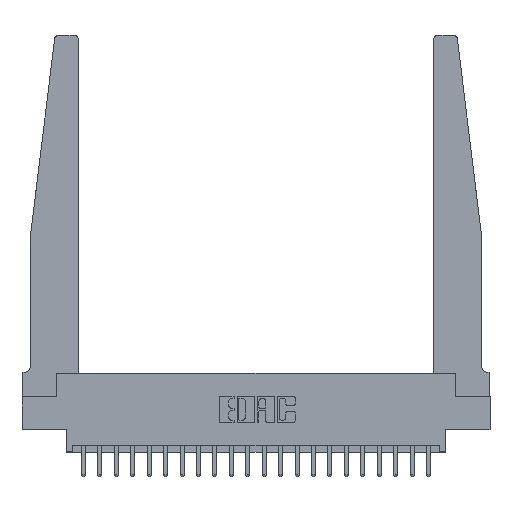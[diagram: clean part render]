
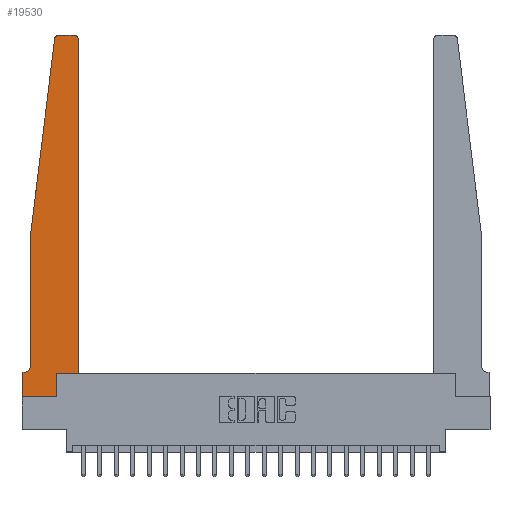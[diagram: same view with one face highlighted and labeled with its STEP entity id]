
A CAD part, top view. The second image highlights one B-rep face of the part: STEP entity #19530.
In plain terms, the highlighted planar face has unit normal (0, 0, 1).
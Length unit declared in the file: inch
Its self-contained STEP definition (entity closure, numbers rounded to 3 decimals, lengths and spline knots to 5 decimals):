
#75 = EDGE_LOOP ( 'NONE', ( #16493, #9969, #19630, #15601, #17411, #15856, #21959, #15008, #15206, #11481, #11396, #4826 ) ) ;
#83 = EDGE_CURVE ( 'NONE', #15609, #19105, #19314, .T. ) ;
#244 = DIRECTION ( 'NONE',  ( 0., 1., 0. ) ) ;
#491 = CIRCLE ( 'NONE', #15062, 0.03 ) ;
#983 = VERTEX_POINT ( 'NONE', #22297 ) ;
#985 = DIRECTION ( 'NONE',  ( -1., 0., 0. ) ) ;
#1679 = VECTOR ( 'NONE', #20016, 39.37008 ) ;
#1795 = DIRECTION ( 'NONE',  ( 1., 0., 0. ) ) ;
#1954 = VECTOR ( 'NONE', #1795, 39.37008 ) ;
#2219 = CARTESIAN_POINT ( 'NONE',  ( 0.2605, 0., 0.37 ) ) ;
#2532 = CARTESIAN_POINT ( 'NONE',  ( 0.065, 1.25, 0.37 ) ) ;
#2690 = CIRCLE ( 'NONE', #9221, 0.05 ) ;
#3061 = CARTESIAN_POINT ( 'NONE',  ( 0., 0., 0.37 ) ) ;
#3669 = CARTESIAN_POINT ( 'NONE',  ( 0.425, 0.18, 0.37 ) ) ;
#4124 = LINE ( 'NONE', #2532, #1679 ) ;
#4391 = DIRECTION ( 'NONE',  ( 0., 0., -1. ) ) ;
#4826 = ORIENTED_EDGE ( 'NONE', *, *, #10889, .T. ) ;
#5089 = CARTESIAN_POINT ( 'NONE',  ( 0., 0., 0.37 ) ) ;
#5115 = LINE ( 'NONE', #3061, #1954 ) ;
#6083 = CARTESIAN_POINT ( 'NONE',  ( 0.425, 0.18, 0.37 ) ) ;
#6183 = DIRECTION ( 'NONE',  ( 1., 0., 0. ) ) ;
#6276 = CARTESIAN_POINT ( 'NONE',  ( 0., 0.1875, 0.37 ) ) ;
#6658 = LINE ( 'NONE', #5089, #7383 ) ;
#6945 = LINE ( 'NONE', #17363, #11354 ) ;
#6952 = EDGE_CURVE ( 'NONE', #21319, #16950, #6658, .T. ) ;
#7167 = CARTESIAN_POINT ( 'NONE',  ( 0.425, 0.18, 0.37 ) ) ;
#7237 = LINE ( 'NONE', #14557, #15813 ) ;
#7383 = VECTOR ( 'NONE', #19022, 39.37008 ) ;
#7424 = VECTOR ( 'NONE', #9434, 39.37008 ) ;
#7453 = CARTESIAN_POINT ( 'NONE',  ( 0.065, 1.25, 0.37 ) ) ;
#7462 = FACE_OUTER_BOUND ( 'NONE', #75, .T. ) ;
#8827 = CARTESIAN_POINT ( 'NONE',  ( 0., 0.1875, 0.37 ) ) ;
#8948 = DIRECTION ( 'NONE',  ( 1., 0., 0. ) ) ;
#9221 = AXIS2_PLACEMENT_3D ( 'NONE', #14782, #4391, #985 ) ;
#9434 = DIRECTION ( 'NONE',  ( 0., 1., 0. ) ) ;
#9969 = ORIENTED_EDGE ( 'NONE', *, *, #12741, .T. ) ;
#10664 = DIRECTION ( 'NONE',  ( 0., 0., 1. ) ) ;
#10825 = DIRECTION ( 'NONE',  ( -1., 0., 0. ) ) ;
#10889 = EDGE_CURVE ( 'NONE', #19105, #20577, #21536, .T. ) ;
#10922 = CARTESIAN_POINT ( 'NONE',  ( 0.065, 0.1875, 0.37 ) ) ;
#11101 = VECTOR ( 'NONE', #244, 39.37008 ) ;
#11354 = VECTOR ( 'NONE', #20872, 39.37008 ) ;
#11396 = ORIENTED_EDGE ( 'NONE', *, *, #83, .T. ) ;
#11481 = ORIENTED_EDGE ( 'NONE', *, *, #11680, .T. ) ;
#11573 = CARTESIAN_POINT ( 'NONE',  ( 0.27653, 2.72, 0.37 ) ) ;
#11680 = EDGE_CURVE ( 'NONE', #983, #15609, #19902, .T. ) ;
#12029 = DIRECTION ( 'NONE',  ( 1., 0., 0. ) ) ;
#12272 = PLANE ( 'NONE',  #13615 ) ;
#12694 = EDGE_CURVE ( 'NONE', #14488, #14847, #2690, .T. ) ;
#12741 = EDGE_CURVE ( 'NONE', #18280, #19455, #491, .T. ) ;
#12948 = VERTEX_POINT ( 'NONE', #7453 ) ;
#12982 = VECTOR ( 'NONE', #6183, 39.37008 ) ;
#13441 = CARTESIAN_POINT ( 'NONE',  ( 0.395, 2.72, 0.37 ) ) ;
#13528 = CARTESIAN_POINT ( 'NONE',  ( 0.24675, 2.72367, 0.37 ) ) ;
#13615 = AXIS2_PLACEMENT_3D ( 'NONE', #8827, #10664, #8948 ) ;
#14480 = CARTESIAN_POINT ( 'NONE',  ( 0.425, 2.72, 0.37 ) ) ;
#14488 = VERTEX_POINT ( 'NONE', #15746 ) ;
#14557 = CARTESIAN_POINT ( 'NONE',  ( 0.065, 1.25, 0.37 ) ) ;
#14782 = CARTESIAN_POINT ( 'NONE',  ( 0.015, 0.2375, 0.37 ) ) ;
#14847 = VERTEX_POINT ( 'NONE', #15197 ) ;
#15008 = ORIENTED_EDGE ( 'NONE', *, *, #19026, .T. ) ;
#15020 = EDGE_CURVE ( 'NONE', #20577, #18280, #6945, .T. ) ;
#15062 = AXIS2_PLACEMENT_3D ( 'NONE', #11573, #15453, #12029 ) ;
#15197 = CARTESIAN_POINT ( 'NONE',  ( 0.015, 0.1875, 0.37 ) ) ;
#15206 = ORIENTED_EDGE ( 'NONE', *, *, #18921, .T. ) ;
#15453 = DIRECTION ( 'NONE',  ( 0., 0., 1. ) ) ;
#15568 = EDGE_CURVE ( 'NONE', #14847, #21319, #19631, .T. ) ;
#15601 = ORIENTED_EDGE ( 'NONE', *, *, #20772, .T. ) ;
#15609 = VERTEX_POINT ( 'NONE', #7167 ) ;
#15746 = CARTESIAN_POINT ( 'NONE',  ( 0.065, 0.2375, 0.37 ) ) ;
#15813 = VECTOR ( 'NONE', #21151, 39.37008 ) ;
#15856 = ORIENTED_EDGE ( 'NONE', *, *, #15568, .T. ) ;
#15947 = CARTESIAN_POINT ( 'NONE',  ( 0., 0., 0.37 ) ) ;
#16493 = ORIENTED_EDGE ( 'NONE', *, *, #15020, .T. ) ;
#16950 = VERTEX_POINT ( 'NONE', #15947 ) ;
#17282 = VECTOR ( 'NONE', #10825, 39.37008 ) ;
#17328 = VERTEX_POINT ( 'NONE', #2219 ) ;
#17363 = CARTESIAN_POINT ( 'NONE',  ( 0.25, 2.75, 0.37 ) ) ;
#17411 = ORIENTED_EDGE ( 'NONE', *, *, #12694, .T. ) ;
#17846 = EDGE_CURVE ( 'NONE', #19455, #12948, #4124, .T. ) ;
#18140 = CARTESIAN_POINT ( 'NONE',  ( 0.395, 2.75, 0.37 ) ) ;
#18280 = VERTEX_POINT ( 'NONE', #20812 ) ;
#18706 = CARTESIAN_POINT ( 'NONE',  ( 0.2605, 0.18, 0.37 ) ) ;
#18921 = EDGE_CURVE ( 'NONE', #17328, #983, #20408, .T. ) ;
#19022 = DIRECTION ( 'NONE',  ( 0., -1., 0. ) ) ;
#19026 = EDGE_CURVE ( 'NONE', #16950, #17328, #5115, .T. ) ;
#19105 = VERTEX_POINT ( 'NONE', #14480 ) ;
#19314 = LINE ( 'NONE', #3669, #11101 ) ;
#19455 = VERTEX_POINT ( 'NONE', #13528 ) ;
#19530 = ADVANCED_FACE ( 'NONE', ( #7462 ), #12272, .T. ) ;
#19630 = ORIENTED_EDGE ( 'NONE', *, *, #17846, .T. ) ;
#19631 = LINE ( 'NONE', #10922, #17282 ) ;
#19902 = LINE ( 'NONE', #6083, #12982 ) ;
#20016 = DIRECTION ( 'NONE',  ( -0.122, -0.992, 0. ) ) ;
#20401 = DIRECTION ( 'NONE',  ( 0., 0., 1. ) ) ;
#20408 = LINE ( 'NONE', #18706, #7424 ) ;
#20577 = VERTEX_POINT ( 'NONE', #18140 ) ;
#20772 = EDGE_CURVE ( 'NONE', #12948, #14488, #7237, .T. ) ;
#20812 = CARTESIAN_POINT ( 'NONE',  ( 0.27653, 2.75, 0.37 ) ) ;
#20872 = DIRECTION ( 'NONE',  ( -1., 0., 0. ) ) ;
#21151 = DIRECTION ( 'NONE',  ( 0., -1., 0. ) ) ;
#21187 = AXIS2_PLACEMENT_3D ( 'NONE', #13441, #20401, #22095 ) ;
#21319 = VERTEX_POINT ( 'NONE', #6276 ) ;
#21536 = CIRCLE ( 'NONE', #21187, 0.03 ) ;
#21959 = ORIENTED_EDGE ( 'NONE', *, *, #6952, .T. ) ;
#22095 = DIRECTION ( 'NONE',  ( 1., 0., 0. ) ) ;
#22297 = CARTESIAN_POINT ( 'NONE',  ( 0.2605, 0.18, 0.37 ) ) ;
